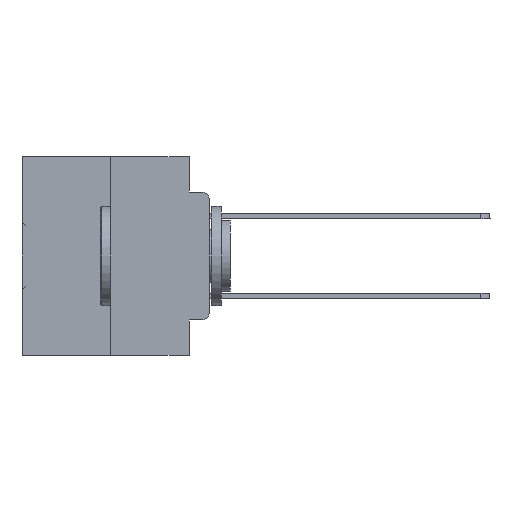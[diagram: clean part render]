
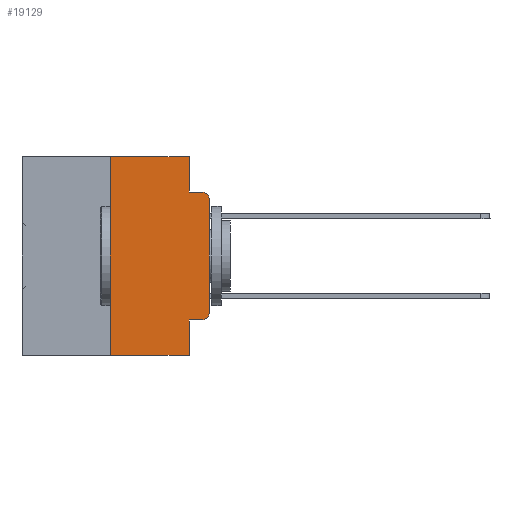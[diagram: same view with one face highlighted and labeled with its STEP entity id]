
A CAD part, left-side view. The second image highlights one B-rep face of the part: STEP entity #19129.
In plain terms, the highlighted planar face has unit normal (-1, 0, 0).
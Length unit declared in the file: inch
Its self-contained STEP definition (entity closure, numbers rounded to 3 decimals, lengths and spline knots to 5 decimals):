
#242 = CARTESIAN_POINT ( 'NONE',  ( 0., 0.25, 0. ) ) ;
#248 = DIRECTION ( 'NONE',  ( 0., 0., -1. ) ) ;
#431 = ORIENTED_EDGE ( 'NONE', *, *, #22523, .F. ) ;
#492 = CARTESIAN_POINT ( 'NONE',  ( 0., 0.051, -0.4115 ) ) ;
#733 = DIRECTION ( 'NONE',  ( 0., -1., 0. ) ) ;
#894 = CIRCLE ( 'NONE', #26345, 0.02 ) ;
#937 = ORIENTED_EDGE ( 'NONE', *, *, #37562, .T. ) ;
#1792 = DIRECTION ( 'NONE',  ( 0., 0., -1. ) ) ;
#2311 = VERTEX_POINT ( 'NONE', #28429 ) ;
#2900 = DIRECTION ( 'NONE',  ( 0., 0., -1. ) ) ;
#3725 = VERTEX_POINT ( 'NONE', #38361 ) ;
#3735 = CARTESIAN_POINT ( 'NONE',  ( 0., 0., -0.3915 ) ) ;
#3746 = CARTESIAN_POINT ( 'NONE',  ( 0., 0.25, 0. ) ) ;
#4077 = EDGE_CURVE ( 'NONE', #7539, #34234, #24335, .T. ) ;
#5474 = DIRECTION ( 'NONE',  ( 1., 0., 0. ) ) ;
#5502 = CARTESIAN_POINT ( 'NONE',  ( 0., 0., 0. ) ) ;
#5508 = VECTOR ( 'NONE', #2900, 39.37008 ) ;
#6188 = LINE ( 'NONE', #11824, #5508 ) ;
#6572 = LINE ( 'NONE', #33381, #11895 ) ;
#6989 = LINE ( 'NONE', #18816, #30986 ) ;
#7539 = VERTEX_POINT ( 'NONE', #9415 ) ;
#7948 = VERTEX_POINT ( 'NONE', #36388 ) ;
#8136 = VECTOR ( 'NONE', #21995, 39.37008 ) ;
#8675 = EDGE_CURVE ( 'NONE', #36894, #22780, #21081, .T. ) ;
#9415 = CARTESIAN_POINT ( 'NONE',  ( 0., 0., -0.1085 ) ) ;
#11194 = EDGE_LOOP ( 'NONE', ( #937, #29747, #14317, #33282, #33978, #431, #24673, #21924, #37720, #17509 ) ) ;
#11687 = CARTESIAN_POINT ( 'NONE',  ( 0., 0.051, -0.5 ) ) ;
#11824 = CARTESIAN_POINT ( 'NONE',  ( 0., 0.051, 0. ) ) ;
#11895 = VECTOR ( 'NONE', #733, 39.37008 ) ;
#12686 = VERTEX_POINT ( 'NONE', #3735 ) ;
#12779 = CARTESIAN_POINT ( 'NONE',  ( 0., 0.051, -0.4115 ) ) ;
#14317 = ORIENTED_EDGE ( 'NONE', *, *, #22306, .F. ) ;
#14384 = PLANE ( 'NONE',  #29725 ) ;
#15596 = VECTOR ( 'NONE', #248, 39.37008 ) ;
#16265 = AXIS2_PLACEMENT_3D ( 'NONE', #16540, #34236, #1792 ) ;
#16540 = CARTESIAN_POINT ( 'NONE',  ( 0., 0.02, -0.1085 ) ) ;
#16659 = CARTESIAN_POINT ( 'NONE',  ( 0., 0.02, -0.3915 ) ) ;
#17317 = DIRECTION ( 'NONE',  ( 0., 0., 1. ) ) ;
#17509 = ORIENTED_EDGE ( 'NONE', *, *, #37075, .T. ) ;
#18816 = CARTESIAN_POINT ( 'NONE',  ( 0., 0.473, 0. ) ) ;
#19129 = ADVANCED_FACE ( 'NONE', ( #32076 ), #14384, .F. ) ;
#19376 = EDGE_CURVE ( 'NONE', #22324, #7948, #6989, .T. ) ;
#20834 = DIRECTION ( 'NONE',  ( 0., -1., 0. ) ) ;
#21081 = LINE ( 'NONE', #492, #34469 ) ;
#21218 = CARTESIAN_POINT ( 'NONE',  ( 0., 0.051, 0. ) ) ;
#21924 = ORIENTED_EDGE ( 'NONE', *, *, #23653, .F. ) ;
#21995 = DIRECTION ( 'NONE',  ( 0., 0., 1. ) ) ;
#22306 = EDGE_CURVE ( 'NONE', #2311, #34234, #26319, .T. ) ;
#22324 = VERTEX_POINT ( 'NONE', #242 ) ;
#22523 = EDGE_CURVE ( 'NONE', #3725, #22324, #36780, .T. ) ;
#22780 = VERTEX_POINT ( 'NONE', #29356 ) ;
#23421 = EDGE_CURVE ( 'NONE', #3725, #27625, #6572, .T. ) ;
#23653 = EDGE_CURVE ( 'NONE', #36894, #27625, #24338, .T. ) ;
#23951 = CARTESIAN_POINT ( 'NONE',  ( 0., 0.051, -0.0885 ) ) ;
#24335 = CIRCLE ( 'NONE', #16265, 0.02 ) ;
#24338 = LINE ( 'NONE', #21218, #15596 ) ;
#24673 = ORIENTED_EDGE ( 'NONE', *, *, #23421, .T. ) ;
#26319 = LINE ( 'NONE', #23951, #27348 ) ;
#26345 = AXIS2_PLACEMENT_3D ( 'NONE', #16659, #28894, #28698 ) ;
#27348 = VECTOR ( 'NONE', #20834, 39.37008 ) ;
#27625 = VERTEX_POINT ( 'NONE', #11687 ) ;
#28190 = EDGE_CURVE ( 'NONE', #7948, #2311, #6188, .T. ) ;
#28429 = CARTESIAN_POINT ( 'NONE',  ( 0., 0.051, -0.0885 ) ) ;
#28698 = DIRECTION ( 'NONE',  ( 0., 0., -1. ) ) ;
#28894 = DIRECTION ( 'NONE',  ( -1., 0., 0. ) ) ;
#29158 = DIRECTION ( 'NONE',  ( 0., 0., -1. ) ) ;
#29187 = LINE ( 'NONE', #5502, #31961 ) ;
#29356 = CARTESIAN_POINT ( 'NONE',  ( 0., 0.02, -0.4115 ) ) ;
#29725 = AXIS2_PLACEMENT_3D ( 'NONE', #32269, #5474, #29158 ) ;
#29747 = ORIENTED_EDGE ( 'NONE', *, *, #4077, .T. ) ;
#30702 = CARTESIAN_POINT ( 'NONE',  ( 0., 0.02, -0.0885 ) ) ;
#30986 = VECTOR ( 'NONE', #36903, 39.37008 ) ;
#31961 = VECTOR ( 'NONE', #17317, 39.37008 ) ;
#32076 = FACE_OUTER_BOUND ( 'NONE', #11194, .T. ) ;
#32269 = CARTESIAN_POINT ( 'NONE',  ( 0., 0.473, 0. ) ) ;
#33282 = ORIENTED_EDGE ( 'NONE', *, *, #28190, .F. ) ;
#33285 = DIRECTION ( 'NONE',  ( 0., -1., 0. ) ) ;
#33381 = CARTESIAN_POINT ( 'NONE',  ( 0., 0.473, -0.5 ) ) ;
#33978 = ORIENTED_EDGE ( 'NONE', *, *, #19376, .F. ) ;
#34234 = VERTEX_POINT ( 'NONE', #30702 ) ;
#34236 = DIRECTION ( 'NONE',  ( -1., 0., 0. ) ) ;
#34469 = VECTOR ( 'NONE', #33285, 39.37008 ) ;
#36388 = CARTESIAN_POINT ( 'NONE',  ( 0., 0.051, 0. ) ) ;
#36780 = LINE ( 'NONE', #3746, #8136 ) ;
#36894 = VERTEX_POINT ( 'NONE', #12779 ) ;
#36903 = DIRECTION ( 'NONE',  ( 0., -1., 0. ) ) ;
#37075 = EDGE_CURVE ( 'NONE', #22780, #12686, #894, .T. ) ;
#37562 = EDGE_CURVE ( 'NONE', #12686, #7539, #29187, .T. ) ;
#37720 = ORIENTED_EDGE ( 'NONE', *, *, #8675, .T. ) ;
#38361 = CARTESIAN_POINT ( 'NONE',  ( 0., 0.25, -0.5 ) ) ;
